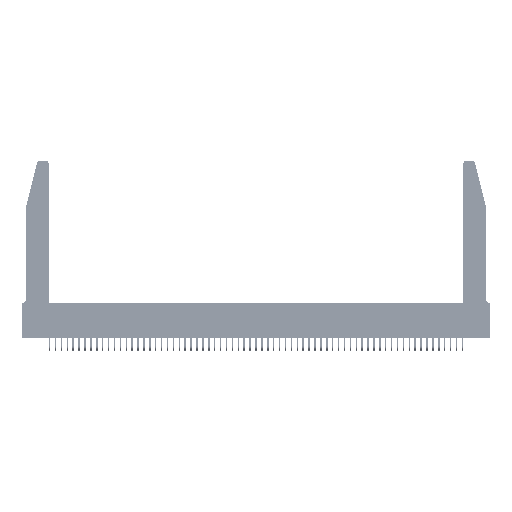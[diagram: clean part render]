
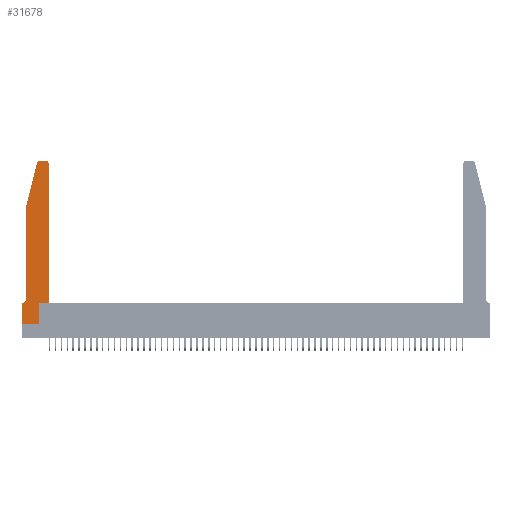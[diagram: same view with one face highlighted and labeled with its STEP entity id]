
A CAD part, top view. The second image highlights one B-rep face of the part: STEP entity #31678.
In plain terms, the highlighted planar face has unit normal (0, 0, 1).
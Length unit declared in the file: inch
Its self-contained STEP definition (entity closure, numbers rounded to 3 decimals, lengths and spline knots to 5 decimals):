
#32 = CARTESIAN_POINT ( 'NONE',  ( 0.284, 2.72, 0.37 ) ) ;
#1307 = EDGE_CURVE ( 'NONE', #56451, #15321, #5610, .T. ) ;
#1862 = CARTESIAN_POINT ( 'NONE',  ( 0.0755, 2., 0.37 ) ) ;
#3753 = DIRECTION ( 'NONE',  ( 0., 0., -1. ) ) ;
#5610 = LINE ( 'NONE', #52435, #45684 ) ;
#5700 = ORIENTED_EDGE ( 'NONE', *, *, #9454, .T. ) ;
#5990 = LINE ( 'NONE', #24533, #34117 ) ;
#7520 = CARTESIAN_POINT ( 'NONE',  ( 0., 0.35, 0.37 ) ) ;
#7917 = EDGE_CURVE ( 'NONE', #21935, #58095, #30053, .T. ) ;
#8312 = EDGE_CURVE ( 'NONE', #29526, #21935, #51252, .T. ) ;
#8315 = DIRECTION ( 'NONE',  ( 1., 0., 0. ) ) ;
#8429 = DIRECTION ( 'NONE',  ( 1., 0., 0. ) ) ;
#8871 = CARTESIAN_POINT ( 'NONE',  ( 0.25487, 2.72718, 0.37 ) ) ;
#9454 = EDGE_CURVE ( 'NONE', #11247, #56451, #25050, .T. ) ;
#10383 = DIRECTION ( 'NONE',  ( -1., 0., 0. ) ) ;
#10594 = CARTESIAN_POINT ( 'NONE',  ( 0.4505, 2.72, 0.37 ) ) ;
#10960 = CARTESIAN_POINT ( 'NONE',  ( 0.2865, 0., 0.37 ) ) ;
#11247 = VERTEX_POINT ( 'NONE', #30647 ) ;
#12745 = CARTESIAN_POINT ( 'NONE',  ( 0.0055, 0.42, 0.37 ) ) ;
#12827 = AXIS2_PLACEMENT_3D ( 'NONE', #12745, #3753, #31423 ) ;
#13455 = CARTESIAN_POINT ( 'NONE',  ( 0.0755, 2., 0.37 ) ) ;
#13480 = VERTEX_POINT ( 'NONE', #47741 ) ;
#13677 = CARTESIAN_POINT ( 'NONE',  ( 0., 0., 0.37 ) ) ;
#13968 = CIRCLE ( 'NONE', #12827, 0.07 ) ;
#14286 = CARTESIAN_POINT ( 'NONE',  ( 0.0755, 0.42, 0.37 ) ) ;
#14328 = LINE ( 'NONE', #27760, #34723 ) ;
#14365 = CARTESIAN_POINT ( 'NONE',  ( 0.0755, 0.35, 0.37 ) ) ;
#14582 = VERTEX_POINT ( 'NONE', #28549 ) ;
#14851 = AXIS2_PLACEMENT_3D ( 'NONE', #22552, #17624, #8429 ) ;
#15321 = VERTEX_POINT ( 'NONE', #10594 ) ;
#15906 = CARTESIAN_POINT ( 'NONE',  ( 0.284, 2.75, 0.37 ) ) ;
#16299 = CARTESIAN_POINT ( 'NONE',  ( 0.0755, 2., 0.37 ) ) ;
#16305 = PLANE ( 'NONE',  #54839 ) ;
#16506 = DIRECTION ( 'NONE',  ( 1., 0., 0. ) ) ;
#17173 = EDGE_CURVE ( 'NONE', #14582, #42036, #23667, .T. ) ;
#17624 = DIRECTION ( 'NONE',  ( 0., 0., 1. ) ) ;
#18402 = VERTEX_POINT ( 'NONE', #14286 ) ;
#18737 = ORIENTED_EDGE ( 'NONE', *, *, #7917, .T. ) ;
#18815 = LINE ( 'NONE', #14365, #34990 ) ;
#20325 = LINE ( 'NONE', #13455, #56927 ) ;
#20577 = EDGE_CURVE ( 'NONE', #15321, #13480, #55115, .T. ) ;
#21935 = VERTEX_POINT ( 'NONE', #8871 ) ;
#22431 = DIRECTION ( 'NONE',  ( 1., 0., 0. ) ) ;
#22552 = CARTESIAN_POINT ( 'NONE',  ( 0.4205, 2.72, 0.37 ) ) ;
#23667 = LINE ( 'NONE', #46672, #32811 ) ;
#23826 = DIRECTION ( 'NONE',  ( -1., 0., 0. ) ) ;
#24533 = CARTESIAN_POINT ( 'NONE',  ( 0.2605, 2.75, 0.37 ) ) ;
#24666 = DIRECTION ( 'NONE',  ( 0., -1., 0. ) ) ;
#25050 = LINE ( 'NONE', #57303, #58154 ) ;
#25475 = FACE_OUTER_BOUND ( 'NONE', #30997, .T. ) ;
#26601 = EDGE_CURVE ( 'NONE', #36542, #11247, #51376, .T. ) ;
#27021 = EDGE_CURVE ( 'NONE', #18402, #34937, #13968, .T. ) ;
#27437 = VECTOR ( 'NONE', #28340, 39.37008 ) ;
#27760 = CARTESIAN_POINT ( 'NONE',  ( 0., 0., 0.37 ) ) ;
#28340 = DIRECTION ( 'NONE',  ( 0., 1., 0. ) ) ;
#28475 = EDGE_CURVE ( 'NONE', #34937, #14582, #18815, .T. ) ;
#28549 = CARTESIAN_POINT ( 'NONE',  ( 0., 0.35, 0.37 ) ) ;
#29526 = VERTEX_POINT ( 'NONE', #15906 ) ;
#30053 = LINE ( 'NONE', #1862, #55494 ) ;
#30172 = EDGE_CURVE ( 'NONE', #13480, #29526, #5990, .T. ) ;
#30647 = CARTESIAN_POINT ( 'NONE',  ( 0.2865, 0.35, 0.37 ) ) ;
#30997 = EDGE_LOOP ( 'NONE', ( #39972, #56482, #18737, #46026, #41500, #52434, #42047, #39050, #57253, #5700, #37066, #33607 ) ) ;
#31423 = DIRECTION ( 'NONE',  ( -1., 0., 0. ) ) ;
#31678 = ADVANCED_FACE ( 'NONE', ( #25475 ), #16305, .T. ) ;
#31835 = DIRECTION ( 'NONE',  ( 1., 0., 0. ) ) ;
#32811 = VECTOR ( 'NONE', #24666, 39.37008 ) ;
#33607 = ORIENTED_EDGE ( 'NONE', *, *, #20577, .T. ) ;
#34117 = VECTOR ( 'NONE', #10383, 39.37008 ) ;
#34711 = DIRECTION ( 'NONE',  ( 0., 1., 0. ) ) ;
#34723 = VECTOR ( 'NONE', #22431, 39.37008 ) ;
#34937 = VERTEX_POINT ( 'NONE', #43923 ) ;
#34990 = VECTOR ( 'NONE', #23826, 39.37008 ) ;
#36542 = VERTEX_POINT ( 'NONE', #10960 ) ;
#37066 = ORIENTED_EDGE ( 'NONE', *, *, #1307, .T. ) ;
#38962 = DIRECTION ( 'NONE',  ( 0., 0., 1. ) ) ;
#39050 = ORIENTED_EDGE ( 'NONE', *, *, #53076, .T. ) ;
#39972 = ORIENTED_EDGE ( 'NONE', *, *, #30172, .T. ) ;
#41500 = ORIENTED_EDGE ( 'NONE', *, *, #27021, .T. ) ;
#41794 = AXIS2_PLACEMENT_3D ( 'NONE', #32, #54102, #31835 ) ;
#42036 = VERTEX_POINT ( 'NONE', #13677 ) ;
#42047 = ORIENTED_EDGE ( 'NONE', *, *, #17173, .T. ) ;
#43671 = CARTESIAN_POINT ( 'NONE',  ( 0.4505, 0.35, 0.37 ) ) ;
#43923 = CARTESIAN_POINT ( 'NONE',  ( 0.0055, 0.35, 0.37 ) ) ;
#45684 = VECTOR ( 'NONE', #34711, 39.37008 ) ;
#46026 = ORIENTED_EDGE ( 'NONE', *, *, #46701, .T. ) ;
#46672 = CARTESIAN_POINT ( 'NONE',  ( 0., 0., 0.37 ) ) ;
#46701 = EDGE_CURVE ( 'NONE', #58095, #18402, #20325, .T. ) ;
#47741 = CARTESIAN_POINT ( 'NONE',  ( 0.4205, 2.75, 0.37 ) ) ;
#50765 = CARTESIAN_POINT ( 'NONE',  ( 0.2865, 0.35, 0.37 ) ) ;
#51252 = CIRCLE ( 'NONE', #41794, 0.03 ) ;
#51376 = LINE ( 'NONE', #50765, #27437 ) ;
#51564 = DIRECTION ( 'NONE',  ( -0.239, -0.971, 0. ) ) ;
#52434 = ORIENTED_EDGE ( 'NONE', *, *, #28475, .T. ) ;
#52435 = CARTESIAN_POINT ( 'NONE',  ( 0.4505, 0.35, 0.37 ) ) ;
#53076 = EDGE_CURVE ( 'NONE', #42036, #36542, #14328, .T. ) ;
#54102 = DIRECTION ( 'NONE',  ( 0., 0., 1. ) ) ;
#54839 = AXIS2_PLACEMENT_3D ( 'NONE', #7520, #38962, #16506 ) ;
#55115 = CIRCLE ( 'NONE', #14851, 0.03 ) ;
#55494 = VECTOR ( 'NONE', #51564, 39.37008 ) ;
#56451 = VERTEX_POINT ( 'NONE', #43671 ) ;
#56482 = ORIENTED_EDGE ( 'NONE', *, *, #8312, .T. ) ;
#56927 = VECTOR ( 'NONE', #57964, 39.37008 ) ;
#57253 = ORIENTED_EDGE ( 'NONE', *, *, #26601, .T. ) ;
#57303 = CARTESIAN_POINT ( 'NONE',  ( 0.4505, 0.35, 0.37 ) ) ;
#57964 = DIRECTION ( 'NONE',  ( 0., -1., 0. ) ) ;
#58095 = VERTEX_POINT ( 'NONE', #16299 ) ;
#58154 = VECTOR ( 'NONE', #8315, 39.37008 ) ;
